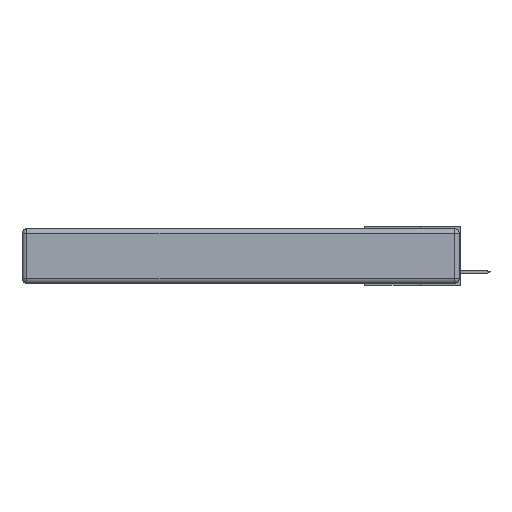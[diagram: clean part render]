
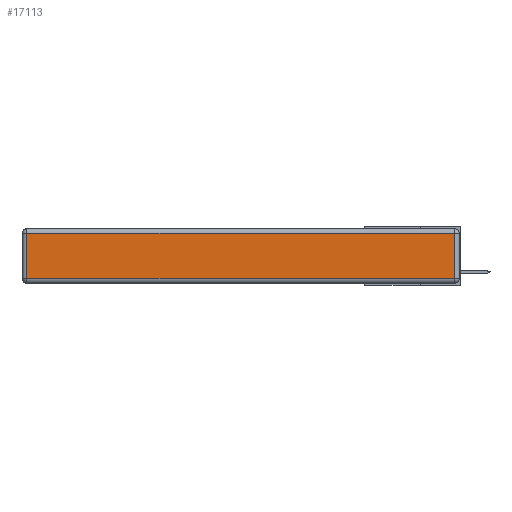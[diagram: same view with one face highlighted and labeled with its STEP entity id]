
A CAD part, left-side view. The second image highlights one B-rep face of the part: STEP entity #17113.
In plain terms, the highlighted planar face has unit normal (-1, 0, 0).
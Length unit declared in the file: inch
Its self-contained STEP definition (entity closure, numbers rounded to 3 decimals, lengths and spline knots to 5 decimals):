
#586 = VERTEX_POINT ( 'NONE', #11222 ) ;
#1054 = DIRECTION ( 'NONE',  ( 0., 1., 0. ) ) ;
#1302 = AXIS2_PLACEMENT_3D ( 'NONE', #16629, #3015, #9101 ) ;
#1832 = EDGE_CURVE ( 'NONE', #8058, #15901, #9697, .T. ) ;
#2383 = VECTOR ( 'NONE', #17943, 39.37008 ) ;
#2559 = CARTESIAN_POINT ( 'NONE',  ( 0., 2.72, -0.03 ) ) ;
#3015 = DIRECTION ( 'NONE',  ( -1., 0., 0. ) ) ;
#4118 = EDGE_CURVE ( 'NONE', #18295, #586, #14695, .T. ) ;
#4860 = ORIENTED_EDGE ( 'NONE', *, *, #1832, .T. ) ;
#5042 = EDGE_LOOP ( 'NONE', ( #17892, #4860, #9158, #19367 ) ) ;
#5702 = FACE_OUTER_BOUND ( 'NONE', #5042, .T. ) ;
#5756 = EDGE_CURVE ( 'NONE', #15901, #18295, #9721, .T. ) ;
#6077 = CARTESIAN_POINT ( 'NONE',  ( 0., 0.03, -0.343 ) ) ;
#6630 = VECTOR ( 'NONE', #17078, 39.37008 ) ;
#8058 = VERTEX_POINT ( 'NONE', #9670 ) ;
#8498 = CARTESIAN_POINT ( 'NONE',  ( 0., 2.72, -0.343 ) ) ;
#8914 = PLANE ( 'NONE',  #1302 ) ;
#9101 = DIRECTION ( 'NONE',  ( 0., 0., 1. ) ) ;
#9158 = ORIENTED_EDGE ( 'NONE', *, *, #5756, .T. ) ;
#9670 = CARTESIAN_POINT ( 'NONE',  ( 0., 0.03, -0.313 ) ) ;
#9697 = LINE ( 'NONE', #6077, #2383 ) ;
#9721 = LINE ( 'NONE', #10257, #11119 ) ;
#10246 = CARTESIAN_POINT ( 'NONE',  ( 0., 0.03, -0.03 ) ) ;
#10257 = CARTESIAN_POINT ( 'NONE',  ( 0., 2.75, -0.03 ) ) ;
#10668 = LINE ( 'NONE', #14018, #6630 ) ;
#11119 = VECTOR ( 'NONE', #1054, 39.37008 ) ;
#11222 = CARTESIAN_POINT ( 'NONE',  ( 0., 2.72, -0.313 ) ) ;
#13053 = VECTOR ( 'NONE', #15947, 39.37008 ) ;
#14018 = CARTESIAN_POINT ( 'NONE',  ( 0., 0., -0.313 ) ) ;
#14695 = LINE ( 'NONE', #8498, #13053 ) ;
#15901 = VERTEX_POINT ( 'NONE', #10246 ) ;
#15947 = DIRECTION ( 'NONE',  ( 0., 0., -1. ) ) ;
#16629 = CARTESIAN_POINT ( 'NONE',  ( 0., 0., -0.343 ) ) ;
#17078 = DIRECTION ( 'NONE',  ( 0., -1., 0. ) ) ;
#17113 = ADVANCED_FACE ( 'NONE', ( #5702 ), #8914, .T. ) ;
#17249 = EDGE_CURVE ( 'NONE', #586, #8058, #10668, .T. ) ;
#17892 = ORIENTED_EDGE ( 'NONE', *, *, #17249, .T. ) ;
#17943 = DIRECTION ( 'NONE',  ( 0., 0., 1. ) ) ;
#18295 = VERTEX_POINT ( 'NONE', #2559 ) ;
#19367 = ORIENTED_EDGE ( 'NONE', *, *, #4118, .T. ) ;
